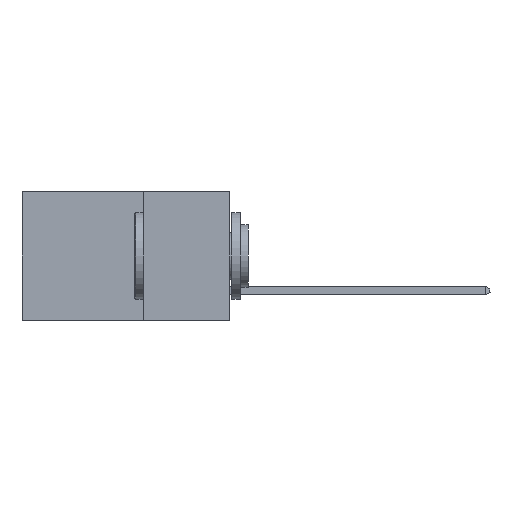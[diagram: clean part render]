
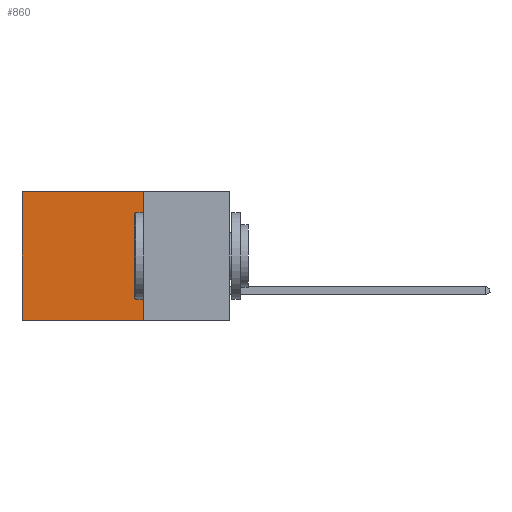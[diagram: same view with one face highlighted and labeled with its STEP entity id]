
A CAD part, left-side view. The second image highlights one B-rep face of the part: STEP entity #860.
In plain terms, the highlighted planar face has unit normal (-1, 0, 0).
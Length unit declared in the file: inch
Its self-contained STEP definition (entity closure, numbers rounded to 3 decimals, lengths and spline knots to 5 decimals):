
#277 = EDGE_CURVE ( 'NONE', #12360, #24658, #5035, .T. ) ;
#860 = ADVANCED_FACE ( 'NONE', ( #21180 ), #1320, .F. ) ;
#1320 = PLANE ( 'NONE',  #22103 ) ;
#3153 = CARTESIAN_POINT ( 'NONE',  ( 0.298, 0.6, 0. ) ) ;
#3965 = VECTOR ( 'NONE', #13792, 39.37008 ) ;
#4203 = EDGE_LOOP ( 'NONE', ( #12291, #7807, #13616, #19156 ) ) ;
#4589 = CARTESIAN_POINT ( 'NONE',  ( 0.298, 0.25, -0.37 ) ) ;
#5035 = LINE ( 'NONE', #19021, #10028 ) ;
#5124 = DIRECTION ( 'NONE',  ( 1., 0., 0. ) ) ;
#5447 = VECTOR ( 'NONE', #20371, 39.37008 ) ;
#6715 = EDGE_CURVE ( 'NONE', #24658, #13317, #23979, .T. ) ;
#7807 = ORIENTED_EDGE ( 'NONE', *, *, #6715, .F. ) ;
#8673 = CARTESIAN_POINT ( 'NONE',  ( 0.298, 0.25, -0.37 ) ) ;
#10028 = VECTOR ( 'NONE', #20671, 39.37008 ) ;
#11423 = LINE ( 'NONE', #23680, #3965 ) ;
#12038 = VERTEX_POINT ( 'NONE', #3153 ) ;
#12291 = ORIENTED_EDGE ( 'NONE', *, *, #13952, .T. ) ;
#12360 = VERTEX_POINT ( 'NONE', #20030 ) ;
#13317 = VERTEX_POINT ( 'NONE', #22245 ) ;
#13616 = ORIENTED_EDGE ( 'NONE', *, *, #277, .F. ) ;
#13792 = DIRECTION ( 'NONE',  ( 0., 1., 0. ) ) ;
#13952 = EDGE_CURVE ( 'NONE', #12038, #13317, #22244, .T. ) ;
#17221 = CARTESIAN_POINT ( 'NONE',  ( 0.298, 0.25, 0. ) ) ;
#18898 = DIRECTION ( 'NONE',  ( 0., 0., -1. ) ) ;
#19021 = CARTESIAN_POINT ( 'NONE',  ( 0.298, 0.25, 0. ) ) ;
#19156 = ORIENTED_EDGE ( 'NONE', *, *, #25420, .T. ) ;
#20030 = CARTESIAN_POINT ( 'NONE',  ( 0.298, 0.25, 0. ) ) ;
#20172 = DIRECTION ( 'NONE',  ( 0., 1., 0. ) ) ;
#20371 = DIRECTION ( 'NONE',  ( 0., 0., -1. ) ) ;
#20612 = CARTESIAN_POINT ( 'NONE',  ( 0.298, 0.6, 0. ) ) ;
#20671 = DIRECTION ( 'NONE',  ( 0., 0., -1. ) ) ;
#20867 = VECTOR ( 'NONE', #20172, 39.37008 ) ;
#21180 = FACE_OUTER_BOUND ( 'NONE', #4203, .T. ) ;
#22103 = AXIS2_PLACEMENT_3D ( 'NONE', #17221, #5124, #18898 ) ;
#22244 = LINE ( 'NONE', #20612, #5447 ) ;
#22245 = CARTESIAN_POINT ( 'NONE',  ( 0.298, 0.6, -0.37 ) ) ;
#23680 = CARTESIAN_POINT ( 'NONE',  ( 0.298, 0.25, 0. ) ) ;
#23979 = LINE ( 'NONE', #4589, #20867 ) ;
#24658 = VERTEX_POINT ( 'NONE', #8673 ) ;
#25420 = EDGE_CURVE ( 'NONE', #12360, #12038, #11423, .T. ) ;
